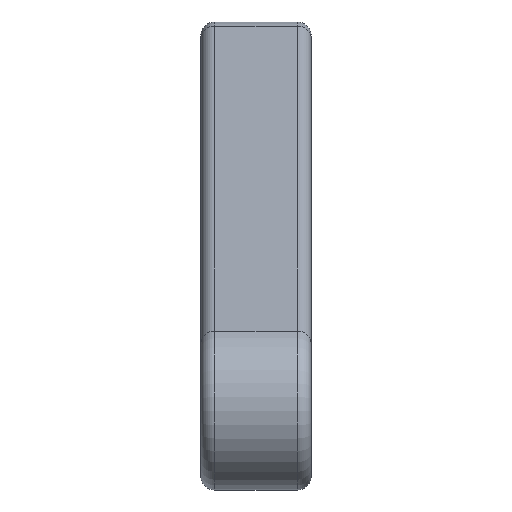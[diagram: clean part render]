
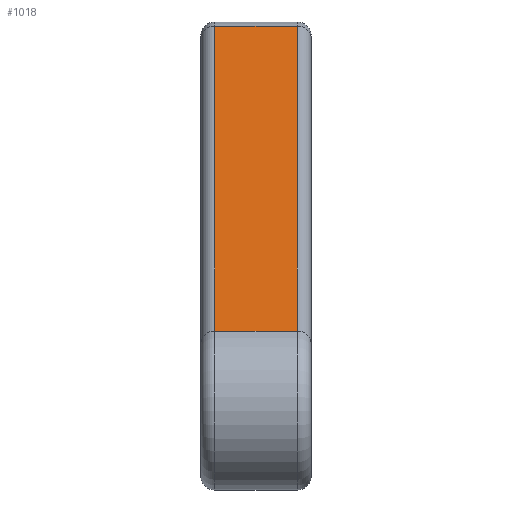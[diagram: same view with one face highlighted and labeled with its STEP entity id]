
A CAD part, front view. The second image highlights one B-rep face of the part: STEP entity #1018.
In plain terms, the highlighted planar face has unit normal (0, -0.438, 0.899).
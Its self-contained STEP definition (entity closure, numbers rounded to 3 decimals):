
#25 = ORIENTED_EDGE ( 'NONE', *, *, #650, .T. ) ;
#48 = LINE ( 'NONE', #604, #150 ) ;
#68 = DIRECTION ( 'NONE',  ( 0., 0.899, 0.438 ) ) ;
#78 = VERTEX_POINT ( 'NONE', #352 ) ;
#119 = LINE ( 'NONE', #1038, #798 ) ;
#125 = EDGE_CURVE ( 'NONE', #380, #1118, #300, .T. ) ;
#150 = VECTOR ( 'NONE', #697, 1000. ) ;
#210 = VECTOR ( 'NONE', #68, 1000. ) ;
#230 = CARTESIAN_POINT ( 'NONE',  ( 3.699, -3.288, 6.741 ) ) ;
#269 = PLANE ( 'NONE',  #740 ) ;
#300 = LINE ( 'NONE', #617, #1033 ) ;
#315 = FACE_OUTER_BOUND ( 'NONE', #443, .T. ) ;
#331 = CARTESIAN_POINT ( 'NONE',  ( 3.699, 52.786, 34.09 ) ) ;
#345 = LINE ( 'NONE', #331, #210 ) ;
#352 = CARTESIAN_POINT ( 'NONE',  ( 3.699, 52.786, 34.09 ) ) ;
#355 = CARTESIAN_POINT ( 'NONE',  ( 4.949, -3.288, 6.741 ) ) ;
#380 = VERTEX_POINT ( 'NONE', #972 ) ;
#437 = DIRECTION ( 'NONE',  ( 0., 0.899, 0.438 ) ) ;
#443 = EDGE_LOOP ( 'NONE', ( #25, #730, #864, #985 ) ) ;
#446 = VERTEX_POINT ( 'NONE', #230 ) ;
#480 = EDGE_CURVE ( 'NONE', #446, #78, #345, .T. ) ;
#490 = CARTESIAN_POINT ( 'NONE',  ( -3.699, -3.288, 6.741 ) ) ;
#521 = DIRECTION ( 'NONE',  ( -1., 0., 0. ) ) ;
#604 = CARTESIAN_POINT ( 'NONE',  ( 4.949, 52.786, 34.09 ) ) ;
#617 = CARTESIAN_POINT ( 'NONE',  ( -3.699, -3.288, 6.741 ) ) ;
#650 = EDGE_CURVE ( 'NONE', #78, #380, #48, .T. ) ;
#664 = EDGE_CURVE ( 'NONE', #446, #1118, #119, .T. ) ;
#678 = DIRECTION ( 'NONE',  ( 0., -0.899, -0.438 ) ) ;
#697 = DIRECTION ( 'NONE',  ( -1., 0., 0. ) ) ;
#730 = ORIENTED_EDGE ( 'NONE', *, *, #125, .T. ) ;
#740 = AXIS2_PLACEMENT_3D ( 'NONE', #355, #962, #437 ) ;
#798 = VECTOR ( 'NONE', #521, 1000. ) ;
#864 = ORIENTED_EDGE ( 'NONE', *, *, #664, .F. ) ;
#962 = DIRECTION ( 'NONE',  ( 0., 0.438, -0.899 ) ) ;
#972 = CARTESIAN_POINT ( 'NONE',  ( -3.699, 52.786, 34.09 ) ) ;
#985 = ORIENTED_EDGE ( 'NONE', *, *, #480, .T. ) ;
#1018 = ADVANCED_FACE ( 'NONE', ( #315 ), #269, .F. ) ;
#1033 = VECTOR ( 'NONE', #678, 1000. ) ;
#1038 = CARTESIAN_POINT ( 'NONE',  ( 4.949, -3.288, 6.741 ) ) ;
#1118 = VERTEX_POINT ( 'NONE', #490 ) ;
